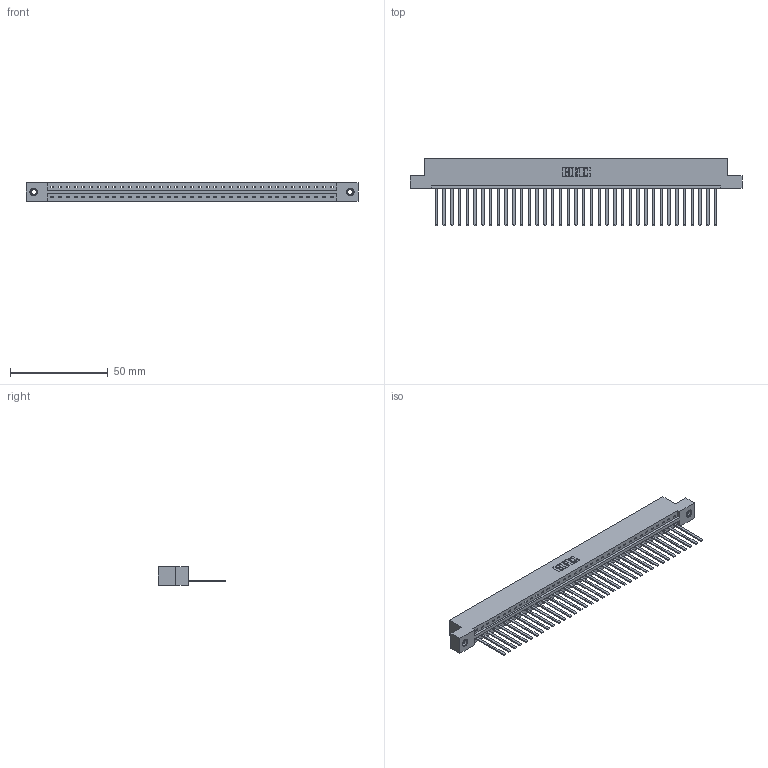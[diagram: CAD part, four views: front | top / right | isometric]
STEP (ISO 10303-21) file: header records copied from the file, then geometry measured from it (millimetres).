
FILE_DESCRIPTION (( 'STEP AP203' ), '1' );
FILE_NAME ('337-037-544-107.STEP', '2019-10-01T15:58:58', ( '' ), ( '' ), 'SwSTEP 2.0', 'SolidWorks 2016', '' );
FILE_SCHEMA (( 'CONFIG_CONTROL_DESIGN' ));
Length unit declared in the file: inch
Products named in the file (4): 337-037-544-107; 345-292-001_345-293-144; 337 Part_Flush Mounting Lugs - 0.156 Dia-TI; 345-250-001_345-250-005-103
Assembly tree (40 placements, depth 2):
  337-037-544-107
    337 Part_Flush Mounting Lugs - 0.156 Dia-TI
    345-292-001_345-293-144  x37
    345-250-001_345-250-005-103  x2
Bounding box: 169.62 x 34.3 x 9.4 mm (x, y, z)
Volume: 17981.7 mm3; surface area: 20004.3 mm2
Topology: 40 solids, 40 shells, 2246 faces, 6737 edges, 4434 vertices
Faces by surface type: plane 1656, cylinder 574, cone 12, torus 4
Entity records: 29152 total; most frequent: CARTESIAN_POINT 5056, ORIENTED_EDGE 5022, DIRECTION 4295, EDGE_CURVE 2511, LINE 2367, VECTOR 2367, VERTEX_POINT 1668, AXIS2_PLACEMENT_3D 964
